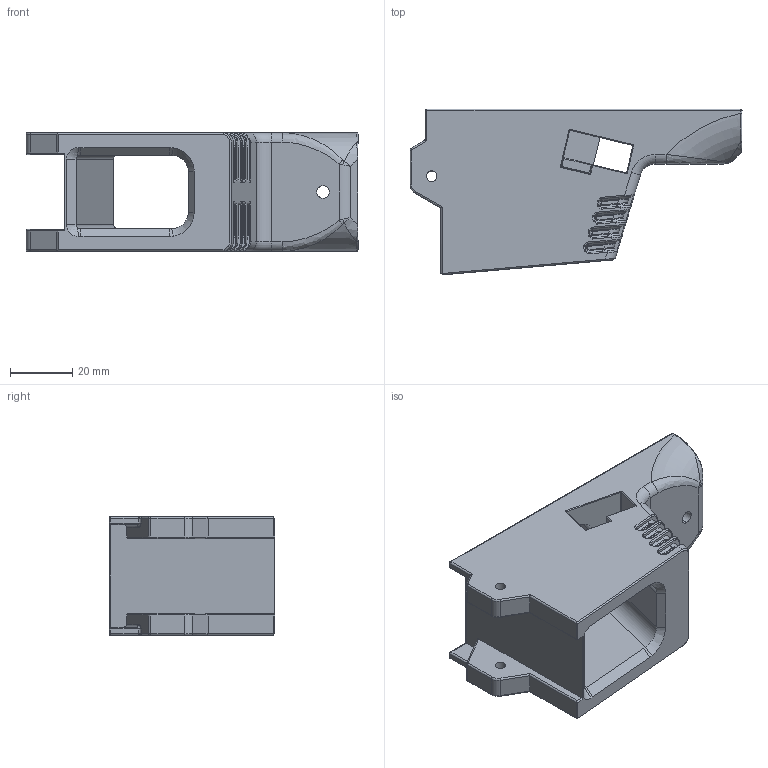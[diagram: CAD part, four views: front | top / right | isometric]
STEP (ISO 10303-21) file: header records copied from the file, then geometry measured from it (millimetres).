
FILE_DESCRIPTION (( 'STEP AP203' ), '1' );
FILE_NAME ('Mag Well Compression Spring.STEP', ( '' ), ( '' ), 'SwSTEP 2.0', 'SolidWorks 2019', '' );
FILE_SCHEMA (( 'CONFIG_CONTROL_DESIGN' ));
Length unit declared in the file: millimetre
Products named in the file (1): Mag Well Compression Spring
Bounding box: 106.51 x 53.17 x 38 mm (x, y, z)
Volume: 86985.9 mm3; surface area: 25035.5 mm2
Topology: 1 solids, 2 shells, 645 faces, 1611 edges, 959 vertices
Faces by surface type: cylinder 253, plane 179, bspline 163, sphere 22, torus 16, cone 12
Entity records: 24471 total; most frequent: CARTESIAN_POINT 10768, ORIENTED_EDGE 3192, DIRECTION 2231, EDGE_CURVE 1596, VERTEX_POINT 954, LINE 807, VECTOR 807, AXIS2_PLACEMENT_3D 712
